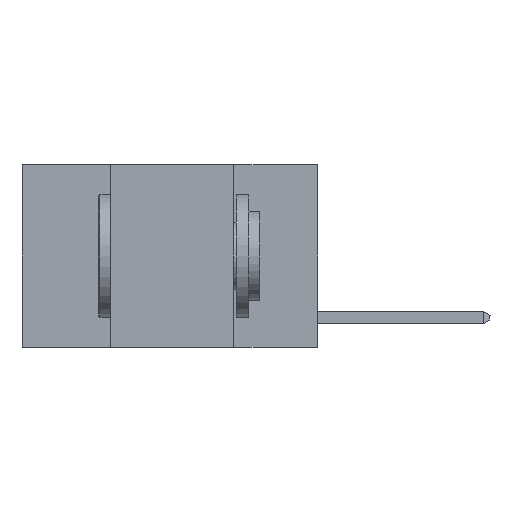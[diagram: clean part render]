
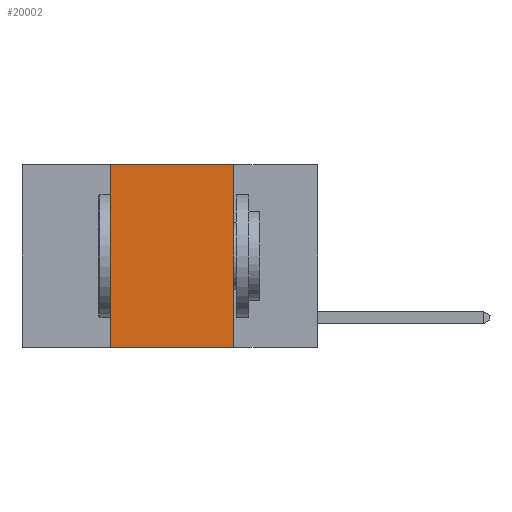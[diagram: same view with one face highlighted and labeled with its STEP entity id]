
A CAD part, left-side view. The second image highlights one B-rep face of the part: STEP entity #20002.
In plain terms, the highlighted planar face has unit normal (-1, 0, 0).
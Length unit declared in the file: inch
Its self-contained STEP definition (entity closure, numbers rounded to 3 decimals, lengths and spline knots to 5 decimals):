
#323 = LINE ( 'NONE', #27620, #6017 ) ;
#1558 = EDGE_CURVE ( 'NONE', #25180, #9600, #4644, .T. ) ;
#2489 = ORIENTED_EDGE ( 'NONE', *, *, #20474, .F. ) ;
#2711 = ORIENTED_EDGE ( 'NONE', *, *, #18607, .F. ) ;
#4644 = LINE ( 'NONE', #18904, #24487 ) ;
#4983 = DIRECTION ( 'NONE',  ( 0., 0., -1. ) ) ;
#6017 = VECTOR ( 'NONE', #9120, 39.37008 ) ;
#7335 = CARTESIAN_POINT ( 'NONE',  ( 0., 0.42, 0. ) ) ;
#7549 = VECTOR ( 'NONE', #4983, 39.37008 ) ;
#7935 = CARTESIAN_POINT ( 'NONE',  ( 0., 0.17, -0.37 ) ) ;
#8261 = AXIS2_PLACEMENT_3D ( 'NONE', #17031, #14815, #21147 ) ;
#9120 = DIRECTION ( 'NONE',  ( 0., 0., 1. ) ) ;
#9243 = ORIENTED_EDGE ( 'NONE', *, *, #1558, .F. ) ;
#9600 = VERTEX_POINT ( 'NONE', #10192 ) ;
#10192 = CARTESIAN_POINT ( 'NONE',  ( 0., 0.17, 0. ) ) ;
#10931 = LINE ( 'NONE', #13580, #7549 ) ;
#11831 = EDGE_LOOP ( 'NONE', ( #2711, #9243, #2489, #26024 ) ) ;
#12148 = EDGE_CURVE ( 'NONE', #18668, #18300, #15139, .T. ) ;
#13102 = VECTOR ( 'NONE', #20564, 39.37008 ) ;
#13580 = CARTESIAN_POINT ( 'NONE',  ( 0., 0.17, 0. ) ) ;
#14815 = DIRECTION ( 'NONE',  ( 1., 0., 0. ) ) ;
#15139 = LINE ( 'NONE', #15838, #13102 ) ;
#15194 = FACE_OUTER_BOUND ( 'NONE', #11831, .T. ) ;
#15838 = CARTESIAN_POINT ( 'NONE',  ( 0., 0.6, -0.37 ) ) ;
#15877 = CARTESIAN_POINT ( 'NONE',  ( 0., 0.42, -0.37 ) ) ;
#16668 = PLANE ( 'NONE',  #8261 ) ;
#17031 = CARTESIAN_POINT ( 'NONE',  ( 0., 0.6, 0. ) ) ;
#18300 = VERTEX_POINT ( 'NONE', #7935 ) ;
#18607 = EDGE_CURVE ( 'NONE', #9600, #18300, #10931, .T. ) ;
#18668 = VERTEX_POINT ( 'NONE', #15877 ) ;
#18904 = CARTESIAN_POINT ( 'NONE',  ( 0., 0.6, 0. ) ) ;
#20002 = ADVANCED_FACE ( 'NONE', ( #15194 ), #16668, .F. ) ;
#20474 = EDGE_CURVE ( 'NONE', #18668, #25180, #323, .T. ) ;
#20564 = DIRECTION ( 'NONE',  ( 0., -1., 0. ) ) ;
#21017 = DIRECTION ( 'NONE',  ( 0., -1., 0. ) ) ;
#21147 = DIRECTION ( 'NONE',  ( 0., 0., -1. ) ) ;
#24487 = VECTOR ( 'NONE', #21017, 39.37008 ) ;
#25180 = VERTEX_POINT ( 'NONE', #7335 ) ;
#26024 = ORIENTED_EDGE ( 'NONE', *, *, #12148, .T. ) ;
#27620 = CARTESIAN_POINT ( 'NONE',  ( 0., 0.42, 0. ) ) ;
